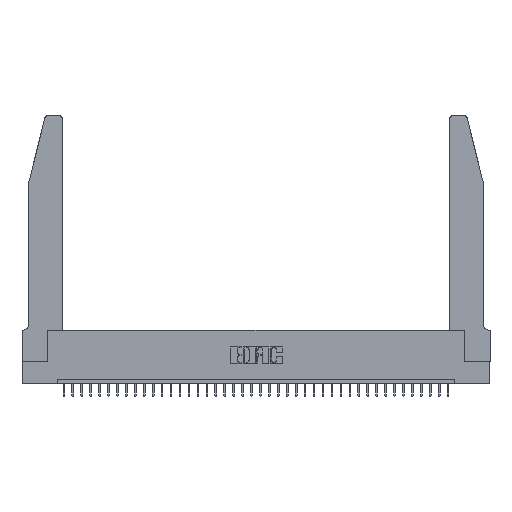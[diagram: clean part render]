
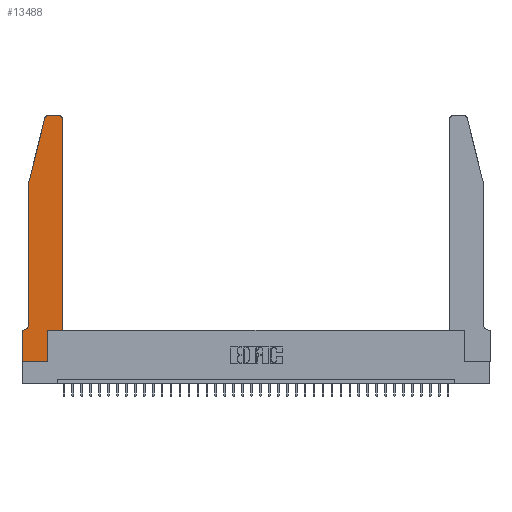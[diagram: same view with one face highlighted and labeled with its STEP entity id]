
A CAD part, top view. The second image highlights one B-rep face of the part: STEP entity #13488.
In plain terms, the highlighted planar face has unit normal (0, 0, 1).
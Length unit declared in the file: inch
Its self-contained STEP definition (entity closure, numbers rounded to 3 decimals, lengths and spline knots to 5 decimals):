
#687 = DIRECTION ( 'NONE',  ( 0., -1., 0. ) ) ;
#729 = VECTOR ( 'NONE', #6663, 39.37008 ) ;
#953 = LINE ( 'NONE', #32982, #7991 ) ;
#3671 = EDGE_CURVE ( 'NONE', #17745, #36907, #5873, .T. ) ;
#4179 = CARTESIAN_POINT ( 'NONE',  ( 0., 0., 0.37 ) ) ;
#4306 = LINE ( 'NONE', #10020, #10853 ) ;
#4859 = ORIENTED_EDGE ( 'NONE', *, *, #23585, .T. ) ;
#5108 = DIRECTION ( 'NONE',  ( -1., 0., 0. ) ) ;
#5684 = CARTESIAN_POINT ( 'NONE',  ( 0.2605, 2.75, 0.37 ) ) ;
#5873 = CIRCLE ( 'NONE', #12547, 0.03 ) ;
#6326 = EDGE_CURVE ( 'NONE', #10830, #28042, #30754, .T. ) ;
#6663 = DIRECTION ( 'NONE',  ( 0., 1., 0. ) ) ;
#6664 = CIRCLE ( 'NONE', #16395, 0.03 ) ;
#7655 = VERTEX_POINT ( 'NONE', #8093 ) ;
#7692 = ORIENTED_EDGE ( 'NONE', *, *, #25775, .T. ) ;
#7773 = LINE ( 'NONE', #31206, #20841 ) ;
#7916 = CARTESIAN_POINT ( 'NONE',  ( 0.0055, 0.35, 0.37 ) ) ;
#7991 = VECTOR ( 'NONE', #10313, 39.37008 ) ;
#8032 = DIRECTION ( 'NONE',  ( 0., 0., 1. ) ) ;
#8093 = CARTESIAN_POINT ( 'NONE',  ( 0.284, 2.75, 0.37 ) ) ;
#8446 = ORIENTED_EDGE ( 'NONE', *, *, #22116, .T. ) ;
#9425 = DIRECTION ( 'NONE',  ( 1., 0., 0. ) ) ;
#10020 = CARTESIAN_POINT ( 'NONE',  ( 0.0755, 2., 0.37 ) ) ;
#10230 = ORIENTED_EDGE ( 'NONE', *, *, #6326, .T. ) ;
#10313 = DIRECTION ( 'NONE',  ( -0.239, -0.971, 0. ) ) ;
#10553 = ORIENTED_EDGE ( 'NONE', *, *, #36602, .T. ) ;
#10830 = VERTEX_POINT ( 'NONE', #33955 ) ;
#10853 = VECTOR ( 'NONE', #687, 39.37008 ) ;
#11193 = CARTESIAN_POINT ( 'NONE',  ( 0.4505, 0.35, 0.37 ) ) ;
#11855 = VECTOR ( 'NONE', #24622, 39.37008 ) ;
#12528 = EDGE_CURVE ( 'NONE', #7655, #36527, #6664, .T. ) ;
#12547 = AXIS2_PLACEMENT_3D ( 'NONE', #33754, #8032, #19654 ) ;
#13468 = FACE_OUTER_BOUND ( 'NONE', #32318, .T. ) ;
#13488 = ADVANCED_FACE ( 'NONE', ( #13468 ), #25070, .T. ) ;
#13549 = DIRECTION ( 'NONE',  ( 0., 1., 0. ) ) ;
#14123 = CARTESIAN_POINT ( 'NONE',  ( 0.0055, 0.42, 0.37 ) ) ;
#14314 = AXIS2_PLACEMENT_3D ( 'NONE', #14123, #34328, #31465 ) ;
#14517 = ORIENTED_EDGE ( 'NONE', *, *, #17613, .T. ) ;
#16057 = EDGE_CURVE ( 'NONE', #36527, #29477, #953, .T. ) ;
#16395 = AXIS2_PLACEMENT_3D ( 'NONE', #20680, #23346, #9425 ) ;
#16438 = CARTESIAN_POINT ( 'NONE',  ( 0., 0., 0.37 ) ) ;
#17305 = CARTESIAN_POINT ( 'NONE',  ( 0.4205, 2.75, 0.37 ) ) ;
#17430 = VECTOR ( 'NONE', #34251, 39.37008 ) ;
#17613 = EDGE_CURVE ( 'NONE', #20060, #26149, #23801, .T. ) ;
#17745 = VERTEX_POINT ( 'NONE', #22067 ) ;
#17965 = EDGE_CURVE ( 'NONE', #28042, #28647, #7773, .T. ) ;
#18451 = CARTESIAN_POINT ( 'NONE',  ( 0.4505, 0.35, 0.37 ) ) ;
#18874 = AXIS2_PLACEMENT_3D ( 'NONE', #36717, #33841, #30034 ) ;
#19654 = DIRECTION ( 'NONE',  ( 1., 0., 0. ) ) ;
#19670 = LINE ( 'NONE', #16438, #11855 ) ;
#20060 = VERTEX_POINT ( 'NONE', #34742 ) ;
#20168 = LINE ( 'NONE', #5684, #20365 ) ;
#20365 = VECTOR ( 'NONE', #34271, 39.37008 ) ;
#20680 = CARTESIAN_POINT ( 'NONE',  ( 0.284, 2.72, 0.37 ) ) ;
#20841 = VECTOR ( 'NONE', #5108, 39.37008 ) ;
#21188 = ORIENTED_EDGE ( 'NONE', *, *, #12528, .T. ) ;
#21376 = LINE ( 'NONE', #36230, #29246 ) ;
#22067 = CARTESIAN_POINT ( 'NONE',  ( 0.4505, 2.72, 0.37 ) ) ;
#22116 = EDGE_CURVE ( 'NONE', #36907, #7655, #20168, .T. ) ;
#23346 = DIRECTION ( 'NONE',  ( 0., 0., 1. ) ) ;
#23443 = ORIENTED_EDGE ( 'NONE', *, *, #17965, .T. ) ;
#23585 = EDGE_CURVE ( 'NONE', #25918, #20060, #19670, .T. ) ;
#23801 = LINE ( 'NONE', #32383, #729 ) ;
#24070 = ORIENTED_EDGE ( 'NONE', *, *, #3671, .T. ) ;
#24267 = CARTESIAN_POINT ( 'NONE',  ( 0., 0., 0.37 ) ) ;
#24622 = DIRECTION ( 'NONE',  ( 1., 0., 0. ) ) ;
#25070 = PLANE ( 'NONE',  #18874 ) ;
#25124 = ORIENTED_EDGE ( 'NONE', *, *, #16057, .T. ) ;
#25338 = VECTOR ( 'NONE', #29536, 39.37008 ) ;
#25547 = VERTEX_POINT ( 'NONE', #18451 ) ;
#25775 = EDGE_CURVE ( 'NONE', #26149, #25547, #26044, .T. ) ;
#25918 = VERTEX_POINT ( 'NONE', #24267 ) ;
#26044 = LINE ( 'NONE', #11193, #17430 ) ;
#26149 = VERTEX_POINT ( 'NONE', #28817 ) ;
#28042 = VERTEX_POINT ( 'NONE', #7916 ) ;
#28647 = VERTEX_POINT ( 'NONE', #35430 ) ;
#28817 = CARTESIAN_POINT ( 'NONE',  ( 0.2865, 0.35, 0.37 ) ) ;
#29196 = EDGE_CURVE ( 'NONE', #29477, #10830, #4306, .T. ) ;
#29246 = VECTOR ( 'NONE', #13549, 39.37008 ) ;
#29477 = VERTEX_POINT ( 'NONE', #35152 ) ;
#29536 = DIRECTION ( 'NONE',  ( 0., -1., 0. ) ) ;
#30034 = DIRECTION ( 'NONE',  ( 1., 0., 0. ) ) ;
#30269 = LINE ( 'NONE', #4179, #25338 ) ;
#30754 = CIRCLE ( 'NONE', #14314, 0.07 ) ;
#31206 = CARTESIAN_POINT ( 'NONE',  ( 0.0755, 0.35, 0.37 ) ) ;
#31465 = DIRECTION ( 'NONE',  ( -1., 0., 0. ) ) ;
#32010 = EDGE_CURVE ( 'NONE', #25547, #17745, #21376, .T. ) ;
#32318 = EDGE_LOOP ( 'NONE', ( #8446, #21188, #25124, #37198, #10230, #23443, #10553, #4859, #14517, #7692, #33786, #24070 ) ) ;
#32383 = CARTESIAN_POINT ( 'NONE',  ( 0.2865, 0.35, 0.37 ) ) ;
#32982 = CARTESIAN_POINT ( 'NONE',  ( 0.0755, 2., 0.37 ) ) ;
#33754 = CARTESIAN_POINT ( 'NONE',  ( 0.4205, 2.72, 0.37 ) ) ;
#33786 = ORIENTED_EDGE ( 'NONE', *, *, #32010, .T. ) ;
#33841 = DIRECTION ( 'NONE',  ( 0., 0., 1. ) ) ;
#33955 = CARTESIAN_POINT ( 'NONE',  ( 0.0755, 0.42, 0.37 ) ) ;
#34251 = DIRECTION ( 'NONE',  ( 1., 0., 0. ) ) ;
#34271 = DIRECTION ( 'NONE',  ( -1., 0., 0. ) ) ;
#34328 = DIRECTION ( 'NONE',  ( 0., 0., -1. ) ) ;
#34704 = CARTESIAN_POINT ( 'NONE',  ( 0.25487, 2.72718, 0.37 ) ) ;
#34742 = CARTESIAN_POINT ( 'NONE',  ( 0.2865, 0., 0.37 ) ) ;
#35152 = CARTESIAN_POINT ( 'NONE',  ( 0.0755, 2., 0.37 ) ) ;
#35430 = CARTESIAN_POINT ( 'NONE',  ( 0., 0.35, 0.37 ) ) ;
#36230 = CARTESIAN_POINT ( 'NONE',  ( 0.4505, 0.35, 0.37 ) ) ;
#36527 = VERTEX_POINT ( 'NONE', #34704 ) ;
#36602 = EDGE_CURVE ( 'NONE', #28647, #25918, #30269, .T. ) ;
#36717 = CARTESIAN_POINT ( 'NONE',  ( 0., 0.35, 0.37 ) ) ;
#36907 = VERTEX_POINT ( 'NONE', #17305 ) ;
#37198 = ORIENTED_EDGE ( 'NONE', *, *, #29196, .T. ) ;
